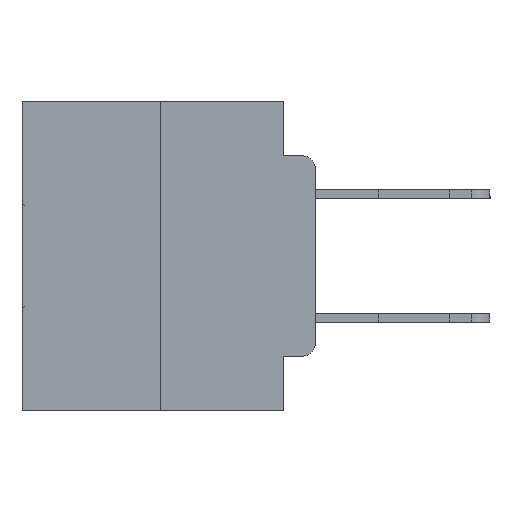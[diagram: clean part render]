
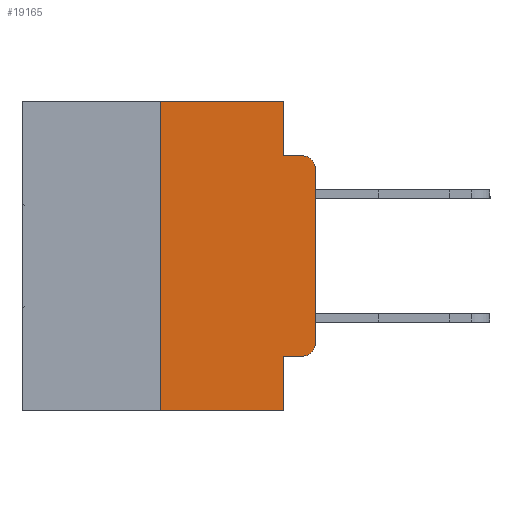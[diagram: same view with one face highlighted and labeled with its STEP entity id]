
A CAD part, left-side view. The second image highlights one B-rep face of the part: STEP entity #19165.
In plain terms, the highlighted planar face has unit normal (-1, 0, 0).
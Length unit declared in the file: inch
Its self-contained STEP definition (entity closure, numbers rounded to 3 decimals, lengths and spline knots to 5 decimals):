
#64 = ORIENTED_EDGE ( 'NONE', *, *, #29771, .T. ) ;
#67 = DIRECTION ( 'NONE',  ( 0., -1., 0. ) ) ;
#751 = LINE ( 'NONE', #31138, #7704 ) ;
#940 = AXIS2_PLACEMENT_3D ( 'NONE', #11598, #28829, #14089 ) ;
#1174 = ORIENTED_EDGE ( 'NONE', *, *, #1607, .F. ) ;
#1510 = VERTEX_POINT ( 'NONE', #19317 ) ;
#1538 = VERTEX_POINT ( 'NONE', #11356 ) ;
#1607 = EDGE_CURVE ( 'NONE', #9482, #17865, #12908, .T. ) ;
#2063 = LINE ( 'NONE', #28915, #28664 ) ;
#2195 = CARTESIAN_POINT ( 'NONE',  ( 0., 0., -0.1085 ) ) ;
#3603 = VERTEX_POINT ( 'NONE', #2195 ) ;
#3631 = DIRECTION ( 'NONE',  ( 0., -1., 0. ) ) ;
#4458 = CARTESIAN_POINT ( 'NONE',  ( 0., 0.473, 0. ) ) ;
#4477 = EDGE_CURVE ( 'NONE', #18351, #1510, #16152, .T. ) ;
#4489 = DIRECTION ( 'NONE',  ( 0., -1., 0. ) ) ;
#5193 = DIRECTION ( 'NONE',  ( 0., 0., 1. ) ) ;
#5449 = ORIENTED_EDGE ( 'NONE', *, *, #9867, .F. ) ;
#6007 = CARTESIAN_POINT ( 'NONE',  ( 0., 0.051, -0.5 ) ) ;
#6415 = ORIENTED_EDGE ( 'NONE', *, *, #4477, .F. ) ;
#6436 = CARTESIAN_POINT ( 'NONE',  ( 0., 0.02, -0.4115 ) ) ;
#6840 = CARTESIAN_POINT ( 'NONE',  ( 0., 0.051, -0.0885 ) ) ;
#7467 = DIRECTION ( 'NONE',  ( 0., 0., -1. ) ) ;
#7704 = VECTOR ( 'NONE', #16423, 39.37008 ) ;
#7715 = EDGE_CURVE ( 'NONE', #22817, #10114, #31556, .T. ) ;
#7865 = CARTESIAN_POINT ( 'NONE',  ( 0., 0.051, -0.4115 ) ) ;
#8268 = LINE ( 'NONE', #12180, #14864 ) ;
#8311 = AXIS2_PLACEMENT_3D ( 'NONE', #28215, #13476, #30667 ) ;
#9019 = VERTEX_POINT ( 'NONE', #6007 ) ;
#9482 = VERTEX_POINT ( 'NONE', #30351 ) ;
#9565 = VECTOR ( 'NONE', #3631, 39.37008 ) ;
#9867 = EDGE_CURVE ( 'NONE', #17865, #21645, #22208, .T. ) ;
#10033 = ORIENTED_EDGE ( 'NONE', *, *, #30978, .T. ) ;
#10114 = VERTEX_POINT ( 'NONE', #10638 ) ;
#10473 = CARTESIAN_POINT ( 'NONE',  ( 0., 0.25, 0. ) ) ;
#10638 = CARTESIAN_POINT ( 'NONE',  ( 0., 0., -0.3915 ) ) ;
#11356 = CARTESIAN_POINT ( 'NONE',  ( 0., 0.051, -0.4115 ) ) ;
#11598 = CARTESIAN_POINT ( 'NONE',  ( 0., 0.02, -0.1085 ) ) ;
#11888 = LINE ( 'NONE', #7865, #32250 ) ;
#12180 = CARTESIAN_POINT ( 'NONE',  ( 0., 0.473, -0.5 ) ) ;
#12406 = CARTESIAN_POINT ( 'NONE',  ( 0., 0.473, 0. ) ) ;
#12908 = LINE ( 'NONE', #10473, #30975 ) ;
#13476 = DIRECTION ( 'NONE',  ( -1., 0., 0. ) ) ;
#14089 = DIRECTION ( 'NONE',  ( 0., 0., -1. ) ) ;
#14186 = DIRECTION ( 'NONE',  ( 0., 0., -1. ) ) ;
#14864 = VECTOR ( 'NONE', #4489, 39.37008 ) ;
#16060 = EDGE_CURVE ( 'NONE', #1538, #22817, #11888, .T. ) ;
#16082 = VECTOR ( 'NONE', #21492, 39.37008 ) ;
#16152 = LINE ( 'NONE', #20952, #9565 ) ;
#16423 = DIRECTION ( 'NONE',  ( 0., 0., 1. ) ) ;
#16650 = CARTESIAN_POINT ( 'NONE',  ( 0., 0.051, 0. ) ) ;
#17865 = VERTEX_POINT ( 'NONE', #32123 ) ;
#18351 = VERTEX_POINT ( 'NONE', #6840 ) ;
#19165 = ADVANCED_FACE ( 'NONE', ( #27542 ), #29637, .F. ) ;
#19317 = CARTESIAN_POINT ( 'NONE',  ( 0., 0.02, -0.0885 ) ) ;
#19682 = CARTESIAN_POINT ( 'NONE',  ( 0., 0.051, 0. ) ) ;
#19898 = EDGE_LOOP ( 'NONE', ( #64, #10033, #6415, #28958, #5449, #1174, #31250, #29491, #31358, #28372 ) ) ;
#20952 = CARTESIAN_POINT ( 'NONE',  ( 0., 0.051, -0.0885 ) ) ;
#21485 = EDGE_CURVE ( 'NONE', #21645, #18351, #2063, .T. ) ;
#21492 = DIRECTION ( 'NONE',  ( 0., 0., -1. ) ) ;
#21645 = VERTEX_POINT ( 'NONE', #19682 ) ;
#22208 = LINE ( 'NONE', #4458, #27998 ) ;
#22323 = DIRECTION ( 'NONE',  ( 1., 0., 0. ) ) ;
#22817 = VERTEX_POINT ( 'NONE', #6436 ) ;
#24664 = CIRCLE ( 'NONE', #940, 0.02 ) ;
#27002 = EDGE_CURVE ( 'NONE', #1538, #9019, #29168, .T. ) ;
#27542 = FACE_OUTER_BOUND ( 'NONE', #19898, .T. ) ;
#27731 = EDGE_CURVE ( 'NONE', #9482, #9019, #8268, .T. ) ;
#27998 = VECTOR ( 'NONE', #31804, 39.37008 ) ;
#28215 = CARTESIAN_POINT ( 'NONE',  ( 0., 0.02, -0.3915 ) ) ;
#28372 = ORIENTED_EDGE ( 'NONE', *, *, #7715, .T. ) ;
#28664 = VECTOR ( 'NONE', #14186, 39.37008 ) ;
#28829 = DIRECTION ( 'NONE',  ( -1., 0., 0. ) ) ;
#28915 = CARTESIAN_POINT ( 'NONE',  ( 0., 0.051, 0. ) ) ;
#28958 = ORIENTED_EDGE ( 'NONE', *, *, #21485, .F. ) ;
#29009 = AXIS2_PLACEMENT_3D ( 'NONE', #12406, #22323, #7467 ) ;
#29168 = LINE ( 'NONE', #16650, #16082 ) ;
#29491 = ORIENTED_EDGE ( 'NONE', *, *, #27002, .F. ) ;
#29637 = PLANE ( 'NONE',  #29009 ) ;
#29771 = EDGE_CURVE ( 'NONE', #10114, #3603, #751, .T. ) ;
#30351 = CARTESIAN_POINT ( 'NONE',  ( 0., 0.25, -0.5 ) ) ;
#30667 = DIRECTION ( 'NONE',  ( 0., 0., -1. ) ) ;
#30975 = VECTOR ( 'NONE', #5193, 39.37008 ) ;
#30978 = EDGE_CURVE ( 'NONE', #3603, #1510, #24664, .T. ) ;
#31138 = CARTESIAN_POINT ( 'NONE',  ( 0., 0., 0. ) ) ;
#31250 = ORIENTED_EDGE ( 'NONE', *, *, #27731, .T. ) ;
#31358 = ORIENTED_EDGE ( 'NONE', *, *, #16060, .T. ) ;
#31556 = CIRCLE ( 'NONE', #8311, 0.02 ) ;
#31804 = DIRECTION ( 'NONE',  ( 0., -1., 0. ) ) ;
#32123 = CARTESIAN_POINT ( 'NONE',  ( 0., 0.25, 0. ) ) ;
#32250 = VECTOR ( 'NONE', #67, 39.37008 ) ;
